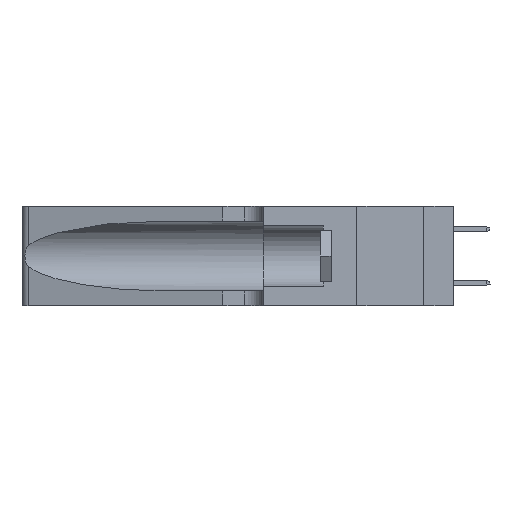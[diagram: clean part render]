
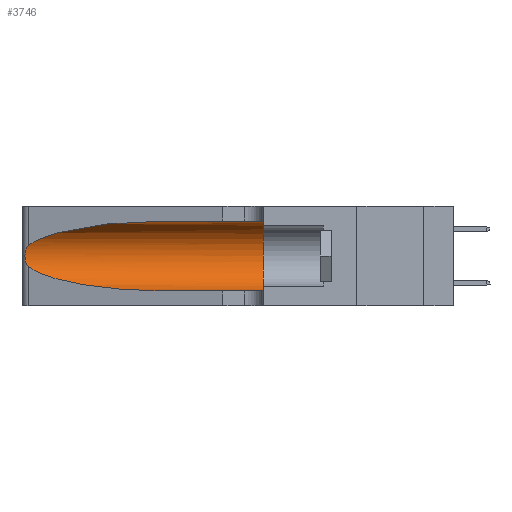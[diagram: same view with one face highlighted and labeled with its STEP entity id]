
A CAD part, left-side view. The second image highlights one B-rep face of the part: STEP entity #3746.
In plain terms, the highlighted cylindrical face has radius 3.308 mm (diameter 6.617 mm), a partial arc.
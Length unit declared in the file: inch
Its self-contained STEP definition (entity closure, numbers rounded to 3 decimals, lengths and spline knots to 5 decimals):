
#322 = VERTEX_POINT ( 'NONE', #23474 ) ;
#559 = FACE_OUTER_BOUND ( 'NONE', #12341, .T. ) ;
#1656 = CARTESIAN_POINT ( 'NONE',  ( 0.2373, 1.15595, 0.28018 ) ) ;
#1780 = CARTESIAN_POINT ( 'NONE',  ( 0.25487, 1.22718, 0.22369 ) ) ;
#2440 = DIRECTION ( 'NONE',  ( 0., -1., 0. ) ) ;
#2691 = DIRECTION ( 'NONE',  ( 0., -1., 0. ) ) ;
#2859 = VERTEX_POINT ( 'NONE', #20946 ) ;
#3053 = DIRECTION ( 'NONE',  ( 0., -1., 0. ) ) ;
#3670 = ORIENTED_EDGE ( 'NONE', *, *, #17473, .F. ) ;
#3712 = CARTESIAN_POINT ( 'NONE',  ( 0.1305, 0.35, 0.31525 ) ) ;
#3744 = CARTESIAN_POINT ( 'NONE',  ( 0.25555, 1.22993, 0.14849 ) ) ;
#3746 = ADVANCED_FACE ( 'NONE', ( #559 ), #18620, .F. ) ;
#3867 = CARTESIAN_POINT ( 'NONE',  ( 0.26017, 1.23833, 0.17102 ) ) ;
#4037 = CARTESIAN_POINT ( 'NONE',  ( 0.1305, 0.35, 0.185 ) ) ;
#4944 = CARTESIAN_POINT ( 'NONE',  ( 0.1305, 1.61858, 0.185 ) ) ;
#5241 = CARTESIAN_POINT ( 'NONE',  ( 0.18966, 0.96281, 0.05475 ) ) ;
#5490 = CARTESIAN_POINT ( 'NONE',  ( 0.2373, 1.15595, 0.08982 ) ) ;
#5898 = VECTOR ( 'NONE', #3053, 39.37008 ) ;
#6665 = VERTEX_POINT ( 'NONE', #9606 ) ;
#7419 = ORIENTED_EDGE ( 'NONE', *, *, #17714, .T. ) ;
#7456 = CARTESIAN_POINT ( 'NONE',  ( 0.25487, 1.22718, 0.22369 ) ) ;
#7957 = EDGE_CURVE ( 'NONE', #8869, #9725, #14472, .T. ) ;
#8047 = VERTEX_POINT ( 'NONE', #12117 ) ;
#8216 = ORIENTED_EDGE ( 'NONE', *, *, #12730, .T. ) ;
#8869 = VERTEX_POINT ( 'NONE', #3712 ) ;
#9304 = CARTESIAN_POINT ( 'NONE',  ( 0.25487, 1.22718, 0.14631 ) ) ;
#9606 = CARTESIAN_POINT ( 'NONE',  ( 0.25487, 1.22718, 0.22369 ) ) ;
#9704 = CARTESIAN_POINT ( 'NONE',  ( 0.25854, 1.2359, 0.20912 ) ) ;
#9725 = VERTEX_POINT ( 'NONE', #10097 ) ;
#9794 = ORIENTED_EDGE ( 'NONE', *, *, #14642, .T. ) ;
#10097 = CARTESIAN_POINT ( 'NONE',  ( 0.1305, 0.35, 0.05475 ) ) ;
#10253 = ORIENTED_EDGE ( 'NONE', *, *, #7957, .F. ) ;
#11727 = CARTESIAN_POINT ( 'NONE',  ( 0.1305, 0.72297, 0.05475 ) ) ;
#11820 = CARTESIAN_POINT ( 'NONE',  ( 0.25555, 1.22994, 0.2215 ) ) ;
#12117 = CARTESIAN_POINT ( 'NONE',  ( 0.1305, 0.72297, 0.31525 ) ) ;
#12341 = EDGE_LOOP ( 'NONE', ( #9794, #7419, #8216, #17374, #10253, #3670 ) ) ;
#12730 = EDGE_CURVE ( 'NONE', #2859, #322, #19385, .T. ) ;
#12887 = DIRECTION ( 'NONE',  ( 0., 0., -1. ) ) ;
#13441 = CARTESIAN_POINT ( 'NONE',  ( 0.18966, 0.96281, 0.31525 ) ) ;
#13535 = CARTESIAN_POINT ( 'NONE',  ( 0.26075, 1.23896, 0.178 ) ) ;
#14472 = CIRCLE ( 'NONE', #17881, 0.13025 ) ;
#14642 = EDGE_CURVE ( 'NONE', #8047, #6665, #20385, .T. ) ;
#15579 = CARTESIAN_POINT ( 'NONE',  ( 0.1305, 0.72297, 0.31525 ) ) ;
#15656 = VECTOR ( 'NONE', #2440, 39.37008 ) ;
#15810 = CARTESIAN_POINT ( 'NONE',  ( 0.25639, 1.23184, 0.21858 ) ) ;
#16500 = CARTESIAN_POINT ( 'NONE',  ( 0.1305, 1.61858, 0.31525 ) ) ;
#16745 = EDGE_CURVE ( 'NONE', #322, #9725, #16990, .T. ) ;
#16990 = LINE ( 'NONE', #24704, #5898 ) ;
#17374 = ORIENTED_EDGE ( 'NONE', *, *, #16745, .T. ) ;
#17473 = EDGE_CURVE ( 'NONE', #8047, #8869, #20624, .T. ) ;
#17702 = B_SPLINE_CURVE_WITH_KNOTS ( 'NONE', 3,
 ( #7456, #11820, #15810, #23539, #9704, #17806, #22060, #13535, #3867, #21807, #21662, #19942, #3744, #9304 ),
 .UNSPECIFIED., .F., .F.,
 ( 4, 2, 2, 2, 2, 2, 4 ),
 ( 0., 0.00027, 0.00053, 0.00107, 0.0016, 0.00187, 0.00214 ),
 .UNSPECIFIED. ) ;
#17714 = EDGE_CURVE ( 'NONE', #6665, #2859, #17702, .T. ) ;
#17806 = CARTESIAN_POINT ( 'NONE',  ( 0.26018, 1.23835, 0.19895 ) ) ;
#17881 = AXIS2_PLACEMENT_3D ( 'NONE', #4037, #23960, #17970 ) ;
#17970 = DIRECTION ( 'NONE',  ( 0., 0., 1. ) ) ;
#18620 = CYLINDRICAL_SURFACE ( 'NONE', #21040, 0.13025 ) ;
#19385 =( BOUNDED_CURVE ( )  B_SPLINE_CURVE ( 3, ( #25682, #5490, #5241, #11727 ),
 .UNSPECIFIED., .F., .T. ) 
 B_SPLINE_CURVE_WITH_KNOTS ( ( 4, 4 ),
 ( 3.44316, 4.71239 ),
 .UNSPECIFIED. ) 
 CURVE ( )  GEOMETRIC_REPRESENTATION_ITEM ( )  RATIONAL_B_SPLINE_CURVE ( ( 1., 0.87, 0.87, 1. ) ) 
 REPRESENTATION_ITEM ( '' )  );
#19942 = CARTESIAN_POINT ( 'NONE',  ( 0.25639, 1.23186, 0.15144 ) ) ;
#20385 =( BOUNDED_CURVE ( )  B_SPLINE_CURVE ( 3, ( #15579, #13441, #1656, #1780 ),
 .UNSPECIFIED., .F., .T. ) 
 B_SPLINE_CURVE_WITH_KNOTS ( ( 4, 4 ),
 ( 1.5708, 2.84003 ),
 .UNSPECIFIED. ) 
 CURVE ( )  GEOMETRIC_REPRESENTATION_ITEM ( )  RATIONAL_B_SPLINE_CURVE ( ( 1., 0.87, 0.87, 1. ) ) 
 REPRESENTATION_ITEM ( '' )  );
#20624 = LINE ( 'NONE', #16500, #15656 ) ;
#20946 = CARTESIAN_POINT ( 'NONE',  ( 0.25487, 1.22718, 0.14631 ) ) ;
#21040 = AXIS2_PLACEMENT_3D ( 'NONE', #4944, #2691, #12887 ) ;
#21662 = CARTESIAN_POINT ( 'NONE',  ( 0.25789, 1.23486, 0.15765 ) ) ;
#21807 = CARTESIAN_POINT ( 'NONE',  ( 0.25856, 1.23593, 0.16098 ) ) ;
#22060 = CARTESIAN_POINT ( 'NONE',  ( 0.26075, 1.23896, 0.19203 ) ) ;
#23474 = CARTESIAN_POINT ( 'NONE',  ( 0.1305, 0.72297, 0.05475 ) ) ;
#23539 = CARTESIAN_POINT ( 'NONE',  ( 0.25787, 1.23484, 0.2124 ) ) ;
#23960 = DIRECTION ( 'NONE',  ( 0., 1., 0. ) ) ;
#24704 = CARTESIAN_POINT ( 'NONE',  ( 0.1305, 1.61858, 0.05475 ) ) ;
#25682 = CARTESIAN_POINT ( 'NONE',  ( 0.25487, 1.22718, 0.14631 ) ) ;
